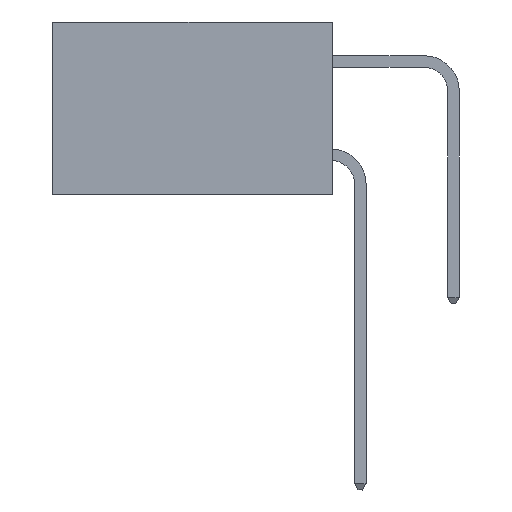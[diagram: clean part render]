
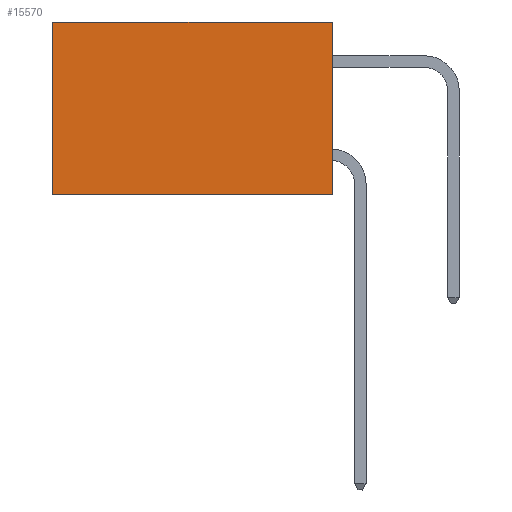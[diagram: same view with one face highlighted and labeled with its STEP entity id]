
A CAD part, left-side view. The second image highlights one B-rep face of the part: STEP entity #15570.
In plain terms, the highlighted planar face has unit normal (-1, 0, 0).
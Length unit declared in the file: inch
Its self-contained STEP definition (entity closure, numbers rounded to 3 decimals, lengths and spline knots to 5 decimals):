
#81 = DIRECTION ( 'NONE',  ( 0., 1., 0. ) ) ;
#1985 = ORIENTED_EDGE ( 'NONE', *, *, #9861, .T. ) ;
#2816 = CARTESIAN_POINT ( 'NONE',  ( 0.298, 0.6, -0.37 ) ) ;
#2985 = CARTESIAN_POINT ( 'NONE',  ( 0.298, 0., -0.37 ) ) ;
#3205 = CARTESIAN_POINT ( 'NONE',  ( 0.298, 0., 0. ) ) ;
#3428 = CARTESIAN_POINT ( 'NONE',  ( 0.298, 0., 0. ) ) ;
#4047 = CARTESIAN_POINT ( 'NONE',  ( 0.298, 0.6, 0. ) ) ;
#4160 = EDGE_CURVE ( 'NONE', #9170, #9112, #11576, .T. ) ;
#4194 = CARTESIAN_POINT ( 'NONE',  ( 0.298, 0.6, 0. ) ) ;
#5143 = CARTESIAN_POINT ( 'NONE',  ( 0.298, 0., 0. ) ) ;
#6547 = EDGE_LOOP ( 'NONE', ( #12267, #7643, #15582, #1985 ) ) ;
#6556 = LINE ( 'NONE', #4194, #8719 ) ;
#6751 = CARTESIAN_POINT ( 'NONE',  ( 0.298, 0., 0. ) ) ;
#7350 = VECTOR ( 'NONE', #81, 39.37008 ) ;
#7351 = PLANE ( 'NONE',  #14739 ) ;
#7521 = DIRECTION ( 'NONE',  ( 0., 0., -1. ) ) ;
#7643 = ORIENTED_EDGE ( 'NONE', *, *, #8528, .F. ) ;
#7892 = VECTOR ( 'NONE', #13182, 39.37008 ) ;
#8528 = EDGE_CURVE ( 'NONE', #9112, #11928, #14460, .T. ) ;
#8719 = VECTOR ( 'NONE', #15413, 39.37008 ) ;
#8720 = FACE_OUTER_BOUND ( 'NONE', #6547, .T. ) ;
#9112 = VERTEX_POINT ( 'NONE', #9771 ) ;
#9170 = VERTEX_POINT ( 'NONE', #6751 ) ;
#9771 = CARTESIAN_POINT ( 'NONE',  ( 0.298, 0., -0.37 ) ) ;
#9861 = EDGE_CURVE ( 'NONE', #9170, #16774, #16066, .T. ) ;
#10069 = DIRECTION ( 'NONE',  ( 1., 0., 0. ) ) ;
#11576 = LINE ( 'NONE', #3428, #7892 ) ;
#11726 = VECTOR ( 'NONE', #14836, 39.37008 ) ;
#11928 = VERTEX_POINT ( 'NONE', #2816 ) ;
#12267 = ORIENTED_EDGE ( 'NONE', *, *, #16259, .T. ) ;
#13182 = DIRECTION ( 'NONE',  ( 0., 0., -1. ) ) ;
#14460 = LINE ( 'NONE', #2985, #7350 ) ;
#14739 = AXIS2_PLACEMENT_3D ( 'NONE', #3205, #10069, #7521 ) ;
#14836 = DIRECTION ( 'NONE',  ( 0., 1., 0. ) ) ;
#15413 = DIRECTION ( 'NONE',  ( 0., 0., -1. ) ) ;
#15570 = ADVANCED_FACE ( 'NONE', ( #8720 ), #7351, .F. ) ;
#15582 = ORIENTED_EDGE ( 'NONE', *, *, #4160, .F. ) ;
#16066 = LINE ( 'NONE', #5143, #11726 ) ;
#16259 = EDGE_CURVE ( 'NONE', #16774, #11928, #6556, .T. ) ;
#16774 = VERTEX_POINT ( 'NONE', #4047 ) ;
